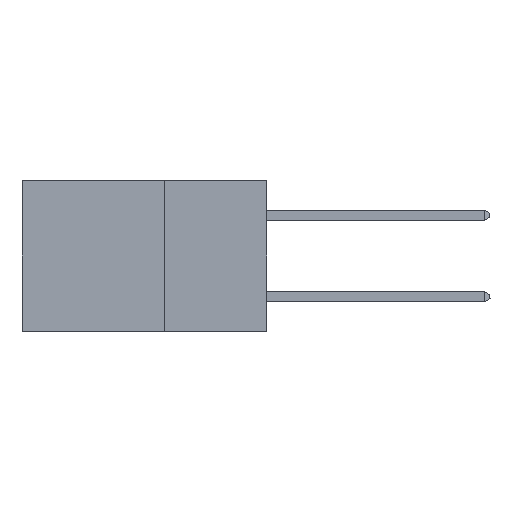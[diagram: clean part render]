
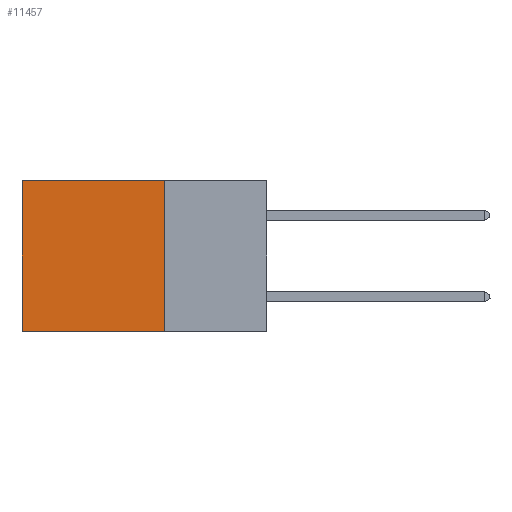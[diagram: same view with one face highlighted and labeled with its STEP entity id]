
A CAD part, left-side view. The second image highlights one B-rep face of the part: STEP entity #11457.
In plain terms, the highlighted planar face has unit normal (-1, 0, 0).
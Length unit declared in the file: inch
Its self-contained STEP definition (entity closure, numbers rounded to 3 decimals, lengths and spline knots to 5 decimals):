
#553 = LINE ( 'NONE', #17580, #7550 ) ;
#1058 = EDGE_CURVE ( 'NONE', #25599, #25807, #553, .T. ) ;
#1270 = CARTESIAN_POINT ( 'NONE',  ( 0.2875, 0.25, 0. ) ) ;
#1524 = EDGE_LOOP ( 'NONE', ( #12359, #24771, #25220, #2080 ) ) ;
#1676 = DIRECTION ( 'NONE',  ( 0., 0., -1. ) ) ;
#2080 = ORIENTED_EDGE ( 'NONE', *, *, #10582, .T. ) ;
#2564 = EDGE_CURVE ( 'NONE', #8437, #23748, #12404, .T. ) ;
#4106 = FACE_OUTER_BOUND ( 'NONE', #1524, .T. ) ;
#5217 = VECTOR ( 'NONE', #23979, 39.37008 ) ;
#6085 = LINE ( 'NONE', #16009, #9426 ) ;
#6283 = EDGE_CURVE ( 'NONE', #23748, #25807, #6085, .T. ) ;
#6700 = LINE ( 'NONE', #13379, #5217 ) ;
#7550 = VECTOR ( 'NONE', #21511, 39.37008 ) ;
#8437 = VERTEX_POINT ( 'NONE', #1270 ) ;
#9426 = VECTOR ( 'NONE', #17977, 39.37008 ) ;
#10328 = CARTESIAN_POINT ( 'NONE',  ( 0.2875, 0.25, 0. ) ) ;
#10582 = EDGE_CURVE ( 'NONE', #8437, #25599, #6700, .T. ) ;
#10774 = DIRECTION ( 'NONE',  ( 1., 0., 0. ) ) ;
#11457 = ADVANCED_FACE ( 'NONE', ( #4106 ), #12325, .F. ) ;
#12325 = PLANE ( 'NONE',  #22966 ) ;
#12359 = ORIENTED_EDGE ( 'NONE', *, *, #1058, .T. ) ;
#12366 = CARTESIAN_POINT ( 'NONE',  ( 0.2875, 0.6, 0. ) ) ;
#12404 = LINE ( 'NONE', #10328, #16203 ) ;
#13379 = CARTESIAN_POINT ( 'NONE',  ( 0.2875, 0.25, 0. ) ) ;
#14539 = DIRECTION ( 'NONE',  ( 0., 0., -1. ) ) ;
#14727 = CARTESIAN_POINT ( 'NONE',  ( 0.2875, 0.6, -0.37 ) ) ;
#16009 = CARTESIAN_POINT ( 'NONE',  ( 0.2875, 0.25, -0.37 ) ) ;
#16203 = VECTOR ( 'NONE', #1676, 39.37008 ) ;
#17580 = CARTESIAN_POINT ( 'NONE',  ( 0.2875, 0.6, 0. ) ) ;
#17977 = DIRECTION ( 'NONE',  ( 0., 1., 0. ) ) ;
#21401 = CARTESIAN_POINT ( 'NONE',  ( 0.2875, 0.25, 0. ) ) ;
#21511 = DIRECTION ( 'NONE',  ( 0., 0., -1. ) ) ;
#22966 = AXIS2_PLACEMENT_3D ( 'NONE', #21401, #10774, #14539 ) ;
#23748 = VERTEX_POINT ( 'NONE', #23970 ) ;
#23970 = CARTESIAN_POINT ( 'NONE',  ( 0.2875, 0.25, -0.37 ) ) ;
#23979 = DIRECTION ( 'NONE',  ( 0., 1., 0. ) ) ;
#24771 = ORIENTED_EDGE ( 'NONE', *, *, #6283, .F. ) ;
#25220 = ORIENTED_EDGE ( 'NONE', *, *, #2564, .F. ) ;
#25599 = VERTEX_POINT ( 'NONE', #12366 ) ;
#25807 = VERTEX_POINT ( 'NONE', #14727 ) ;
